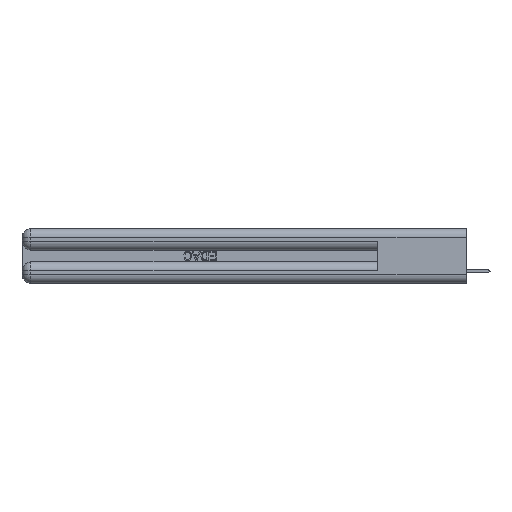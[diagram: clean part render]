
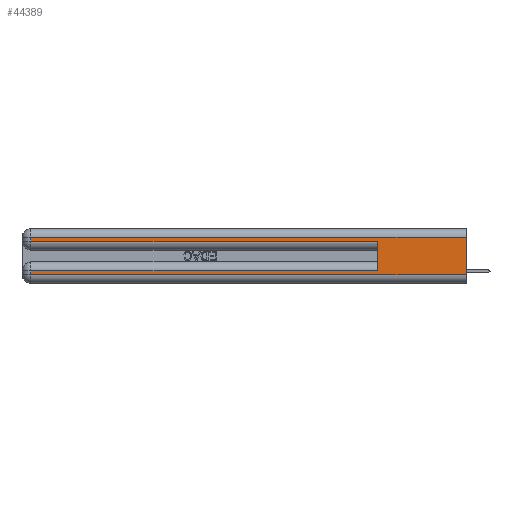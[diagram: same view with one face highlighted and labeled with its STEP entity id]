
A CAD part, left-side view. The second image highlights one B-rep face of the part: STEP entity #44389.
In plain terms, the highlighted planar face has unit normal (-1, 0, 0).
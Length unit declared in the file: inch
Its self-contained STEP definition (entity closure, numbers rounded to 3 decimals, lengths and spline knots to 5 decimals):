
#1000 = VERTEX_POINT ( 'NONE', #45008 ) ;
#1650 = DIRECTION ( 'NONE',  ( 0., 0., -1. ) ) ;
#1773 = LINE ( 'NONE', #37767, #6835 ) ;
#2614 = LINE ( 'NONE', #35229, #26252 ) ;
#3602 = EDGE_CURVE ( 'NONE', #1000, #30245, #4365, .T. ) ;
#4100 = VECTOR ( 'NONE', #24048, 39.37008 ) ;
#4365 = LINE ( 'NONE', #23225, #13312 ) ;
#4674 = VERTEX_POINT ( 'NONE', #27477 ) ;
#5009 = CARTESIAN_POINT ( 'NONE',  ( 0., 0., 0.285 ) ) ;
#5256 = ORIENTED_EDGE ( 'NONE', *, *, #3602, .T. ) ;
#5363 = CARTESIAN_POINT ( 'NONE',  ( 0., 0.6, 0.285 ) ) ;
#6074 = VERTEX_POINT ( 'NONE', #7643 ) ;
#6261 = DIRECTION ( 'NONE',  ( 0., 0., -1. ) ) ;
#6543 = DIRECTION ( 'NONE',  ( 0., 1., 0. ) ) ;
#6722 = DIRECTION ( 'NONE',  ( 1., 0., 0. ) ) ;
#6741 = EDGE_CURVE ( 'NONE', #34677, #43219, #32103, .T. ) ;
#6835 = VECTOR ( 'NONE', #16637, 39.37008 ) ;
#6887 = VERTEX_POINT ( 'NONE', #46234 ) ;
#7643 = CARTESIAN_POINT ( 'NONE',  ( 0., 2.94, 0.31 ) ) ;
#8573 = ORIENTED_EDGE ( 'NONE', *, *, #23935, .T. ) ;
#8856 = ORIENTED_EDGE ( 'NONE', *, *, #12853, .F. ) ;
#10751 = CARTESIAN_POINT ( 'NONE',  ( 0., 0., 0.37 ) ) ;
#11187 = DIRECTION ( 'NONE',  ( 0., 0., 1. ) ) ;
#11269 = EDGE_CURVE ( 'NONE', #6074, #34677, #40703, .T. ) ;
#12517 = CARTESIAN_POINT ( 'NONE',  ( 0., 2.94, 0.06 ) ) ;
#12718 = FACE_OUTER_BOUND ( 'NONE', #32294, .T. ) ;
#12853 = EDGE_CURVE ( 'NONE', #6887, #43219, #22680, .T. ) ;
#13312 = VECTOR ( 'NONE', #1650, 39.37008 ) ;
#13540 = LINE ( 'NONE', #10751, #44093 ) ;
#15803 = DIRECTION ( 'NONE',  ( 0., -1., 0. ) ) ;
#16467 = VECTOR ( 'NONE', #11187, 39.37008 ) ;
#16633 = CARTESIAN_POINT ( 'NONE',  ( 0., 2.94, 0.37 ) ) ;
#16637 = DIRECTION ( 'NONE',  ( 0., 1., 0. ) ) ;
#18434 = DIRECTION ( 'NONE',  ( 0., 0., -1. ) ) ;
#18658 = VECTOR ( 'NONE', #32415, 39.37008 ) ;
#20721 = EDGE_CURVE ( 'NONE', #41247, #6074, #2614, .T. ) ;
#20790 = ORIENTED_EDGE ( 'NONE', *, *, #20721, .T. ) ;
#21396 = CARTESIAN_POINT ( 'NONE',  ( 0., 0., 0.06 ) ) ;
#22470 = VECTOR ( 'NONE', #15803, 39.37008 ) ;
#22680 = LINE ( 'NONE', #29053, #16467 ) ;
#22892 = CARTESIAN_POINT ( 'NONE',  ( 0., 2.94, 0.285 ) ) ;
#23225 = CARTESIAN_POINT ( 'NONE',  ( 0., 2.94, 0.37 ) ) ;
#23675 = ORIENTED_EDGE ( 'NONE', *, *, #46171, .T. ) ;
#23935 = EDGE_CURVE ( 'NONE', #30245, #4674, #44667, .T. ) ;
#24048 = DIRECTION ( 'NONE',  ( 0., 0., -1. ) ) ;
#24397 = AXIS2_PLACEMENT_3D ( 'NONE', #24693, #6722, #6261 ) ;
#24693 = CARTESIAN_POINT ( 'NONE',  ( 0., 0., 0.37 ) ) ;
#26225 = ORIENTED_EDGE ( 'NONE', *, *, #6741, .T. ) ;
#26252 = VECTOR ( 'NONE', #6543, 39.37008 ) ;
#27477 = CARTESIAN_POINT ( 'NONE',  ( 0., 0., 0.06 ) ) ;
#29053 = CARTESIAN_POINT ( 'NONE',  ( 0., 0.6, 0.145 ) ) ;
#30245 = VERTEX_POINT ( 'NONE', #12517 ) ;
#32103 = LINE ( 'NONE', #5009, #22470 ) ;
#32294 = EDGE_LOOP ( 'NONE', ( #38548, #20790, #44255, #26225, #8856, #23675, #5256, #8573 ) ) ;
#32415 = DIRECTION ( 'NONE',  ( 0., -1., 0. ) ) ;
#34463 = PLANE ( 'NONE',  #24397 ) ;
#34677 = VERTEX_POINT ( 'NONE', #22892 ) ;
#35229 = CARTESIAN_POINT ( 'NONE',  ( 0., 0., 0.31 ) ) ;
#37767 = CARTESIAN_POINT ( 'NONE',  ( 0., 0., 0.085 ) ) ;
#38548 = ORIENTED_EDGE ( 'NONE', *, *, #42241, .F. ) ;
#40703 = LINE ( 'NONE', #16633, #4100 ) ;
#41247 = VERTEX_POINT ( 'NONE', #41927 ) ;
#41927 = CARTESIAN_POINT ( 'NONE',  ( 0., 0., 0.31 ) ) ;
#42241 = EDGE_CURVE ( 'NONE', #41247, #4674, #13540, .T. ) ;
#43219 = VERTEX_POINT ( 'NONE', #5363 ) ;
#44093 = VECTOR ( 'NONE', #18434, 39.37008 ) ;
#44255 = ORIENTED_EDGE ( 'NONE', *, *, #11269, .T. ) ;
#44389 = ADVANCED_FACE ( 'NONE', ( #12718 ), #34463, .F. ) ;
#44667 = LINE ( 'NONE', #21396, #18658 ) ;
#45008 = CARTESIAN_POINT ( 'NONE',  ( 0., 2.94, 0.085 ) ) ;
#46171 = EDGE_CURVE ( 'NONE', #6887, #1000, #1773, .T. ) ;
#46234 = CARTESIAN_POINT ( 'NONE',  ( 0., 0.6, 0.085 ) ) ;
